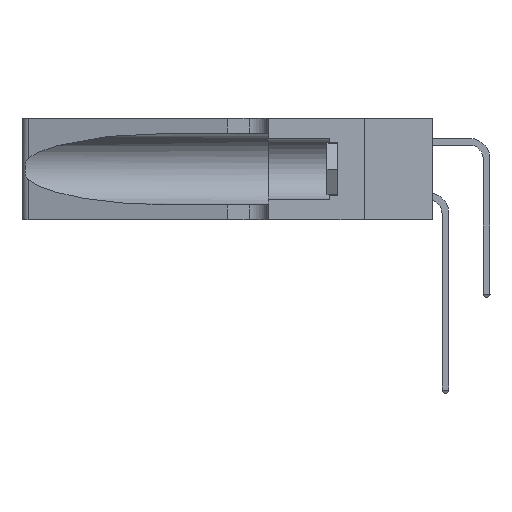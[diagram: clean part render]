
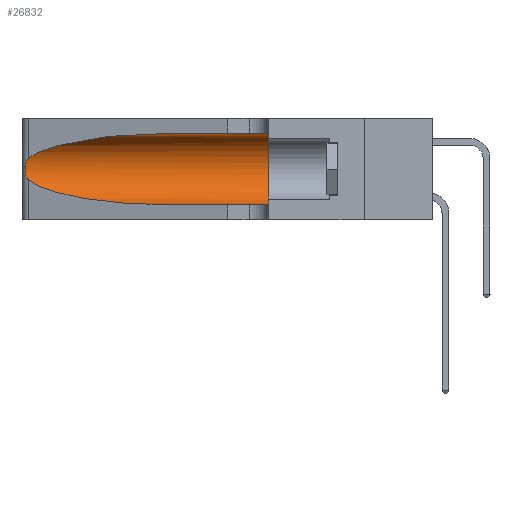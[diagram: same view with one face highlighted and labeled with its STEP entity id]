
A CAD part, left-side view. The second image highlights one B-rep face of the part: STEP entity #26832.
In plain terms, the highlighted cylindrical face has radius 3.308 mm (diameter 6.617 mm), a partial arc.
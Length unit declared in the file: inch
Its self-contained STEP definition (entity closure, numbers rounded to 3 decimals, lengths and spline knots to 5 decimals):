
#139 = VERTEX_POINT ( 'NONE', #25148 ) ;
#2087 = FACE_OUTER_BOUND ( 'NONE', #9742, .T. ) ;
#3016 = CARTESIAN_POINT ( 'NONE',  ( 0.25856, 1.23593, 0.16098 ) ) ;
#3232 = CARTESIAN_POINT ( 'NONE',  ( 0.1305, 1.61858, 0.31525 ) ) ;
#4372 = CARTESIAN_POINT ( 'NONE',  ( 0.1305, 0.72297, 0.05475 ) ) ;
#6016 = CARTESIAN_POINT ( 'NONE',  ( 0.2373, 1.15595, 0.28018 ) ) ;
#6365 = CARTESIAN_POINT ( 'NONE',  ( 0.25639, 1.23186, 0.15144 ) ) ;
#8345 = LINE ( 'NONE', #32825, #41678 ) ;
#9163 = VERTEX_POINT ( 'NONE', #21282 ) ;
#9540 = CARTESIAN_POINT ( 'NONE',  ( 0.25555, 1.22994, 0.2215 ) ) ;
#9541 = AXIS2_PLACEMENT_3D ( 'NONE', #12942, #35538, #16204 ) ;
#9680 = CARTESIAN_POINT ( 'NONE',  ( 0.25487, 1.22718, 0.14631 ) ) ;
#9742 = EDGE_LOOP ( 'NONE', ( #17958, #11922, #13044, #25316, #27293, #28264 ) ) ;
#9773 = VERTEX_POINT ( 'NONE', #30376 ) ;
#9885 = B_SPLINE_CURVE_WITH_KNOTS ( 'NONE', 3,
 ( #12652, #9540, #12792, #35381, #16070, #38605, #19349, #41827, #22595, #3016, #25813, #6365, #29076, #9680 ),
 .UNSPECIFIED., .F., .F.,
 ( 4, 2, 2, 2, 2, 2, 4 ),
 ( 0., 0.00027, 0.00053, 0.00107, 0.0016, 0.00187, 0.00214 ),
 .UNSPECIFIED. ) ;
#10684 = EDGE_CURVE ( 'NONE', #9773, #35129, #9885, .T. ) ;
#10881 = CARTESIAN_POINT ( 'NONE',  ( 0.2373, 1.15595, 0.08982 ) ) ;
#11512 = EDGE_CURVE ( 'NONE', #35129, #9163, #29326, .T. ) ;
#11922 = ORIENTED_EDGE ( 'NONE', *, *, #10684, .T. ) ;
#12652 = CARTESIAN_POINT ( 'NONE',  ( 0.25487, 1.22718, 0.22369 ) ) ;
#12792 = CARTESIAN_POINT ( 'NONE',  ( 0.25639, 1.23184, 0.21858 ) ) ;
#12942 = CARTESIAN_POINT ( 'NONE',  ( 0.1305, 1.61858, 0.185 ) ) ;
#13044 = ORIENTED_EDGE ( 'NONE', *, *, #11512, .T. ) ;
#14777 = LINE ( 'NONE', #3232, #16824 ) ;
#15861 = CARTESIAN_POINT ( 'NONE',  ( 0.1305, 0.35, 0.185 ) ) ;
#16070 = CARTESIAN_POINT ( 'NONE',  ( 0.25854, 1.2359, 0.20912 ) ) ;
#16204 = DIRECTION ( 'NONE',  ( 0., 0., -1. ) ) ;
#16794 = EDGE_CURVE ( 'NONE', #139, #9773, #41152, .T. ) ;
#16824 = VECTOR ( 'NONE', #26038, 39.37008 ) ;
#17428 = CARTESIAN_POINT ( 'NONE',  ( 0.25487, 1.22718, 0.14631 ) ) ;
#17756 = VERTEX_POINT ( 'NONE', #40710 ) ;
#17958 = ORIENTED_EDGE ( 'NONE', *, *, #16794, .T. ) ;
#18828 = VERTEX_POINT ( 'NONE', #39227 ) ;
#18873 = CIRCLE ( 'NONE', #30519, 0.13025 ) ;
#19156 = DIRECTION ( 'NONE',  ( 0., 0., 1. ) ) ;
#19349 = CARTESIAN_POINT ( 'NONE',  ( 0.26075, 1.23896, 0.19203 ) ) ;
#21282 = CARTESIAN_POINT ( 'NONE',  ( 0.1305, 0.72297, 0.05475 ) ) ;
#21707 = EDGE_CURVE ( 'NONE', #17756, #18828, #18873, .T. ) ;
#21796 = EDGE_CURVE ( 'NONE', #139, #17756, #14777, .T. ) ;
#22264 = CARTESIAN_POINT ( 'NONE',  ( 0.1305, 0.72297, 0.31525 ) ) ;
#22595 = CARTESIAN_POINT ( 'NONE',  ( 0.26017, 1.23833, 0.17102 ) ) ;
#23907 = CARTESIAN_POINT ( 'NONE',  ( 0.18966, 0.96281, 0.05475 ) ) ;
#25148 = CARTESIAN_POINT ( 'NONE',  ( 0.1305, 0.72297, 0.31525 ) ) ;
#25316 = ORIENTED_EDGE ( 'NONE', *, *, #35479, .T. ) ;
#25813 = CARTESIAN_POINT ( 'NONE',  ( 0.25789, 1.23486, 0.15765 ) ) ;
#26038 = DIRECTION ( 'NONE',  ( 0., -1., 0. ) ) ;
#26832 = ADVANCED_FACE ( 'NONE', ( #2087 ), #27070, .F. ) ;
#27070 = CYLINDRICAL_SURFACE ( 'NONE', #9541, 0.13025 ) ;
#27293 = ORIENTED_EDGE ( 'NONE', *, *, #21707, .F. ) ;
#27342 = CARTESIAN_POINT ( 'NONE',  ( 0.25487, 1.22718, 0.14631 ) ) ;
#28264 = ORIENTED_EDGE ( 'NONE', *, *, #21796, .F. ) ;
#28737 = CARTESIAN_POINT ( 'NONE',  ( 0.25487, 1.22718, 0.22369 ) ) ;
#29076 = CARTESIAN_POINT ( 'NONE',  ( 0.25555, 1.22993, 0.14849 ) ) ;
#29326 =( BOUNDED_CURVE ( )  B_SPLINE_CURVE ( 3, ( #17428, #10881, #23907, #4372 ),
 .UNSPECIFIED., .F., .F. ) 
 B_SPLINE_CURVE_WITH_KNOTS ( ( 4, 4 ),
 ( 3.44316, 4.71239 ),
 .UNSPECIFIED. ) 
 CURVE ( )  GEOMETRIC_REPRESENTATION_ITEM ( )  RATIONAL_B_SPLINE_CURVE ( ( 1., 0.87, 0.87, 1. ) ) 
 REPRESENTATION_ITEM ( '' )  );
#30376 = CARTESIAN_POINT ( 'NONE',  ( 0.25487, 1.22718, 0.22369 ) ) ;
#30519 = AXIS2_PLACEMENT_3D ( 'NONE', #15861, #38398, #19156 ) ;
#32825 = CARTESIAN_POINT ( 'NONE',  ( 0.1305, 1.61858, 0.05475 ) ) ;
#35129 = VERTEX_POINT ( 'NONE', #27342 ) ;
#35381 = CARTESIAN_POINT ( 'NONE',  ( 0.25787, 1.23484, 0.2124 ) ) ;
#35479 = EDGE_CURVE ( 'NONE', #9163, #18828, #8345, .T. ) ;
#35538 = DIRECTION ( 'NONE',  ( 0., -1., 0. ) ) ;
#36045 = DIRECTION ( 'NONE',  ( 0., -1., 0. ) ) ;
#38398 = DIRECTION ( 'NONE',  ( 0., 1., 0. ) ) ;
#38605 = CARTESIAN_POINT ( 'NONE',  ( 0.26018, 1.23835, 0.19895 ) ) ;
#39227 = CARTESIAN_POINT ( 'NONE',  ( 0.1305, 0.35, 0.05475 ) ) ;
#40710 = CARTESIAN_POINT ( 'NONE',  ( 0.1305, 0.35, 0.31525 ) ) ;
#41152 =( BOUNDED_CURVE ( )  B_SPLINE_CURVE ( 3, ( #22264, #41492, #6016, #28737 ),
 .UNSPECIFIED., .F., .F. ) 
 B_SPLINE_CURVE_WITH_KNOTS ( ( 4, 4 ),
 ( 1.5708, 2.84003 ),
 .UNSPECIFIED. ) 
 CURVE ( )  GEOMETRIC_REPRESENTATION_ITEM ( )  RATIONAL_B_SPLINE_CURVE ( ( 1., 0.87, 0.87, 1. ) ) 
 REPRESENTATION_ITEM ( '' )  );
#41492 = CARTESIAN_POINT ( 'NONE',  ( 0.18966, 0.96281, 0.31525 ) ) ;
#41678 = VECTOR ( 'NONE', #36045, 39.37008 ) ;
#41827 = CARTESIAN_POINT ( 'NONE',  ( 0.26075, 1.23896, 0.178 ) ) ;
